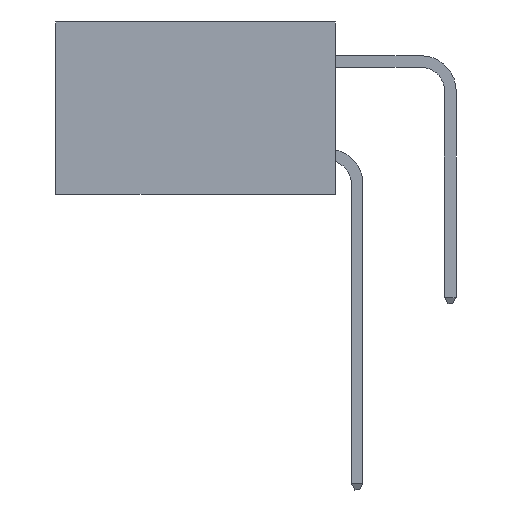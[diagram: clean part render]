
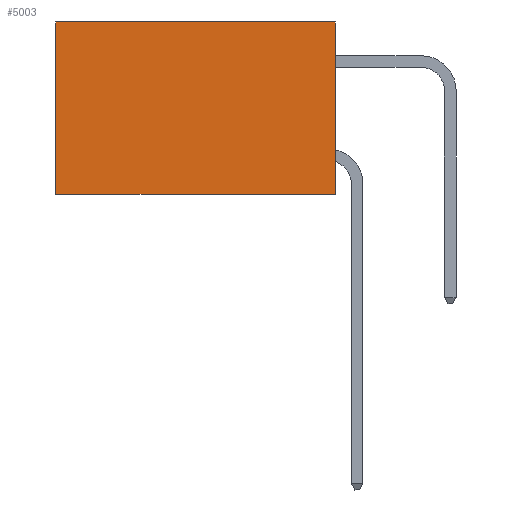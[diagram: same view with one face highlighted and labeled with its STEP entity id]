
A CAD part, left-side view. The second image highlights one B-rep face of the part: STEP entity #5003.
In plain terms, the highlighted planar face has unit normal (-1, 0, 0).
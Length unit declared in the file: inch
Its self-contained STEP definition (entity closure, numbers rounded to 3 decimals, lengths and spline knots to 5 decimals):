
#636 = CARTESIAN_POINT ( 'NONE',  ( 0.2875, 0., 0. ) ) ;
#1071 = PLANE ( 'NONE',  #12132 ) ;
#1215 = DIRECTION ( 'NONE',  ( 0., 1., 0. ) ) ;
#2120 = CARTESIAN_POINT ( 'NONE',  ( 0.2875, 0., 0. ) ) ;
#2432 = ORIENTED_EDGE ( 'NONE', *, *, #11642, .F. ) ;
#2534 = FACE_OUTER_BOUND ( 'NONE', #8022, .T. ) ;
#2867 = DIRECTION ( 'NONE',  ( 1., 0., 0. ) ) ;
#4271 = LINE ( 'NONE', #9739, #8542 ) ;
#4463 = EDGE_CURVE ( 'NONE', #15279, #5561, #4271, .T. ) ;
#4486 = VECTOR ( 'NONE', #6639, 39.37008 ) ;
#5003 = ADVANCED_FACE ( 'NONE', ( #2534 ), #1071, .F. ) ;
#5069 = LINE ( 'NONE', #15608, #4486 ) ;
#5561 = VERTEX_POINT ( 'NONE', #20864 ) ;
#6154 = DIRECTION ( 'NONE',  ( 0., 0., -1. ) ) ;
#6639 = DIRECTION ( 'NONE',  ( 0., 0., -1. ) ) ;
#7834 = EDGE_CURVE ( 'NONE', #15279, #16246, #12922, .T. ) ;
#8022 = EDGE_LOOP ( 'NONE', ( #10277, #2432, #14231, #17889 ) ) ;
#8542 = VECTOR ( 'NONE', #6154, 39.37008 ) ;
#8945 = VECTOR ( 'NONE', #1215, 39.37008 ) ;
#9687 = DIRECTION ( 'NONE',  ( 0., 1., 0. ) ) ;
#9739 = CARTESIAN_POINT ( 'NONE',  ( 0.2875, 0., 0. ) ) ;
#10277 = ORIENTED_EDGE ( 'NONE', *, *, #15443, .T. ) ;
#11642 = EDGE_CURVE ( 'NONE', #5561, #21628, #13755, .T. ) ;
#12132 = AXIS2_PLACEMENT_3D ( 'NONE', #13753, #2867, #15518 ) ;
#12922 = LINE ( 'NONE', #636, #17046 ) ;
#13487 = CARTESIAN_POINT ( 'NONE',  ( 0.2875, 0.6, -0.37 ) ) ;
#13753 = CARTESIAN_POINT ( 'NONE',  ( 0.2875, 0., 0. ) ) ;
#13755 = LINE ( 'NONE', #15656, #8945 ) ;
#14231 = ORIENTED_EDGE ( 'NONE', *, *, #4463, .F. ) ;
#15279 = VERTEX_POINT ( 'NONE', #2120 ) ;
#15443 = EDGE_CURVE ( 'NONE', #16246, #21628, #5069, .T. ) ;
#15518 = DIRECTION ( 'NONE',  ( 0., 0., -1. ) ) ;
#15608 = CARTESIAN_POINT ( 'NONE',  ( 0.2875, 0.6, 0. ) ) ;
#15656 = CARTESIAN_POINT ( 'NONE',  ( 0.2875, 0., -0.37 ) ) ;
#16169 = CARTESIAN_POINT ( 'NONE',  ( 0.2875, 0.6, 0. ) ) ;
#16246 = VERTEX_POINT ( 'NONE', #16169 ) ;
#17046 = VECTOR ( 'NONE', #9687, 39.37008 ) ;
#17889 = ORIENTED_EDGE ( 'NONE', *, *, #7834, .T. ) ;
#20864 = CARTESIAN_POINT ( 'NONE',  ( 0.2875, 0., -0.37 ) ) ;
#21628 = VERTEX_POINT ( 'NONE', #13487 ) ;
